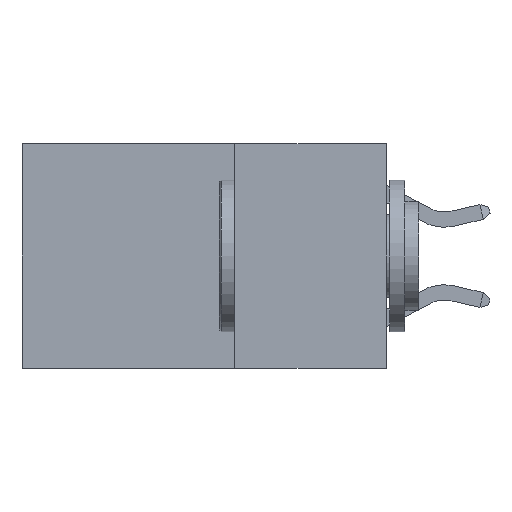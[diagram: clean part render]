
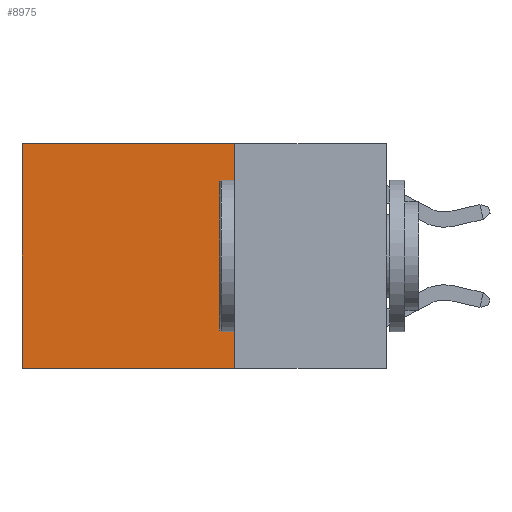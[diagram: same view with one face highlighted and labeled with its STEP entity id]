
A CAD part, left-side view. The second image highlights one B-rep face of the part: STEP entity #8975.
In plain terms, the highlighted planar face has unit normal (-1, 0, 0).
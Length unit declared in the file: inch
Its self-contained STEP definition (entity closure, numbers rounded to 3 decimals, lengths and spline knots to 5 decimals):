
#23 = ORIENTED_EDGE ( 'NONE', *, *, #6393, .F. ) ;
#118 = DIRECTION ( 'NONE',  ( 0., 0., -1. ) ) ;
#167 = CARTESIAN_POINT ( 'NONE',  ( 0.2625, 0.25, 0. ) ) ;
#477 = PLANE ( 'NONE',  #5951 ) ;
#628 = FACE_OUTER_BOUND ( 'NONE', #6565, .T. ) ;
#632 = VECTOR ( 'NONE', #118, 39.37008 ) ;
#779 = LINE ( 'NONE', #10484, #5163 ) ;
#799 = DIRECTION ( 'NONE',  ( 0., 1., 0. ) ) ;
#1212 = VERTEX_POINT ( 'NONE', #8454 ) ;
#1335 = DIRECTION ( 'NONE',  ( 1., 0., 0. ) ) ;
#1608 = CARTESIAN_POINT ( 'NONE',  ( 0.2625, 0.25, 0. ) ) ;
#1652 = DIRECTION ( 'NONE',  ( 0., 1., 0. ) ) ;
#2469 = CARTESIAN_POINT ( 'NONE',  ( 0.2625, 0.6, -0.37 ) ) ;
#2476 = VERTEX_POINT ( 'NONE', #7784 ) ;
#2938 = LINE ( 'NONE', #167, #632 ) ;
#3638 = EDGE_CURVE ( 'NONE', #6505, #2476, #2938, .T. ) ;
#4418 = ORIENTED_EDGE ( 'NONE', *, *, #5997, .T. ) ;
#4513 = VECTOR ( 'NONE', #7664, 39.37008 ) ;
#5163 = VECTOR ( 'NONE', #799, 39.37008 ) ;
#5230 = ORIENTED_EDGE ( 'NONE', *, *, #3638, .F. ) ;
#5396 = EDGE_CURVE ( 'NONE', #6505, #1212, #6826, .T. ) ;
#5951 = AXIS2_PLACEMENT_3D ( 'NONE', #8096, #1335, #7356 ) ;
#5997 = EDGE_CURVE ( 'NONE', #1212, #7648, #8777, .T. ) ;
#6393 = EDGE_CURVE ( 'NONE', #2476, #7648, #779, .T. ) ;
#6505 = VERTEX_POINT ( 'NONE', #9399 ) ;
#6565 = EDGE_LOOP ( 'NONE', ( #4418, #23, #5230, #8000 ) ) ;
#6826 = LINE ( 'NONE', #1608, #8817 ) ;
#6914 = CARTESIAN_POINT ( 'NONE',  ( 0.2625, 0.6, 0. ) ) ;
#7356 = DIRECTION ( 'NONE',  ( 0., 0., -1. ) ) ;
#7648 = VERTEX_POINT ( 'NONE', #2469 ) ;
#7664 = DIRECTION ( 'NONE',  ( 0., 0., -1. ) ) ;
#7784 = CARTESIAN_POINT ( 'NONE',  ( 0.2625, 0.25, -0.37 ) ) ;
#8000 = ORIENTED_EDGE ( 'NONE', *, *, #5396, .T. ) ;
#8096 = CARTESIAN_POINT ( 'NONE',  ( 0.2625, 0.25, 0. ) ) ;
#8454 = CARTESIAN_POINT ( 'NONE',  ( 0.2625, 0.6, 0. ) ) ;
#8777 = LINE ( 'NONE', #6914, #4513 ) ;
#8817 = VECTOR ( 'NONE', #1652, 39.37008 ) ;
#8975 = ADVANCED_FACE ( 'NONE', ( #628 ), #477, .F. ) ;
#9399 = CARTESIAN_POINT ( 'NONE',  ( 0.2625, 0.25, 0. ) ) ;
#10484 = CARTESIAN_POINT ( 'NONE',  ( 0.2625, 0.25, -0.37 ) ) ;
